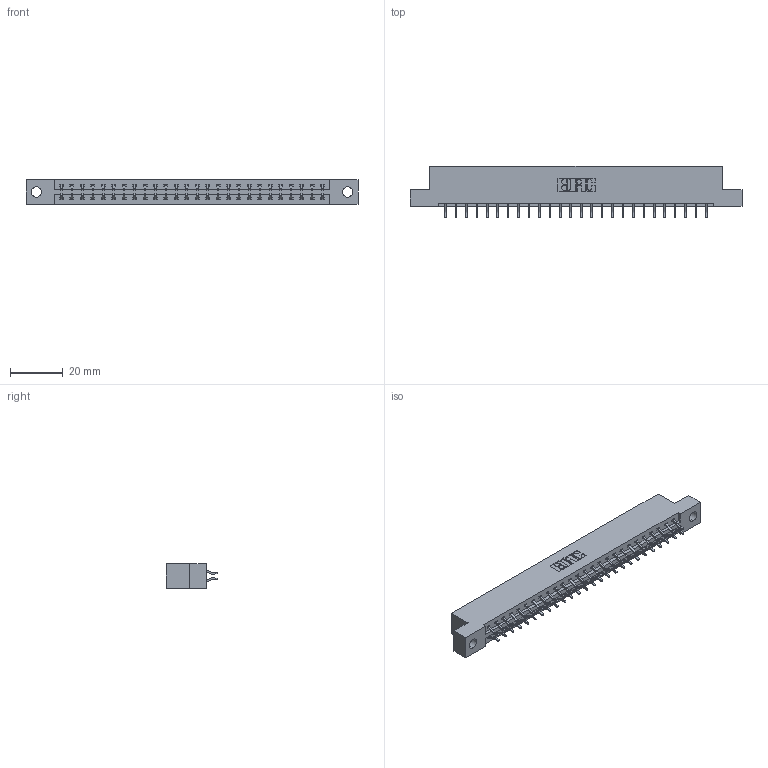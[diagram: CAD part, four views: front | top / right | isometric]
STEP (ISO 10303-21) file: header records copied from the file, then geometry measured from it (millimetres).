
FILE_DESCRIPTION (( 'STEP AP203' ), '1' );
FILE_NAME ('337-052-556-204.STEP', '2018-08-09T23:23:26', ( '' ), ( '' ), 'SwSTEP 2.0', 'SolidWorks 2016', '' );
FILE_SCHEMA (( 'CONFIG_CONTROL_DESIGN' ));
Length unit declared in the file: inch
Products named in the file (3): 337 Part_Flush Mounting Lugs - 0.156 Dia-TH; 345-292-001_556 Tail; 337-052-556-204
Assembly tree (53 placements, depth 2):
  337-052-556-204
    337 Part_Flush Mounting Lugs - 0.156 Dia-TH
    345-292-001_556 Tail  x52
Bounding box: 126.03 x 19.57 x 9.4 mm (x, y, z)
Volume: 12979.7 mm3; surface area: 14260.6 mm2
Topology: 53 solids, 53 shells, 3234 faces, 9619 edges, 6342 vertices
Faces by surface type: plane 2254, cylinder 980
Entity records: 22451 total; most frequent: CARTESIAN_POINT 3810, ORIENTED_EDGE 3734, DIRECTION 3259, EDGE_CURVE 1867, LINE 1731, VECTOR 1731, VERTEX_POINT 1242, AXIS2_PLACEMENT_3D 764
